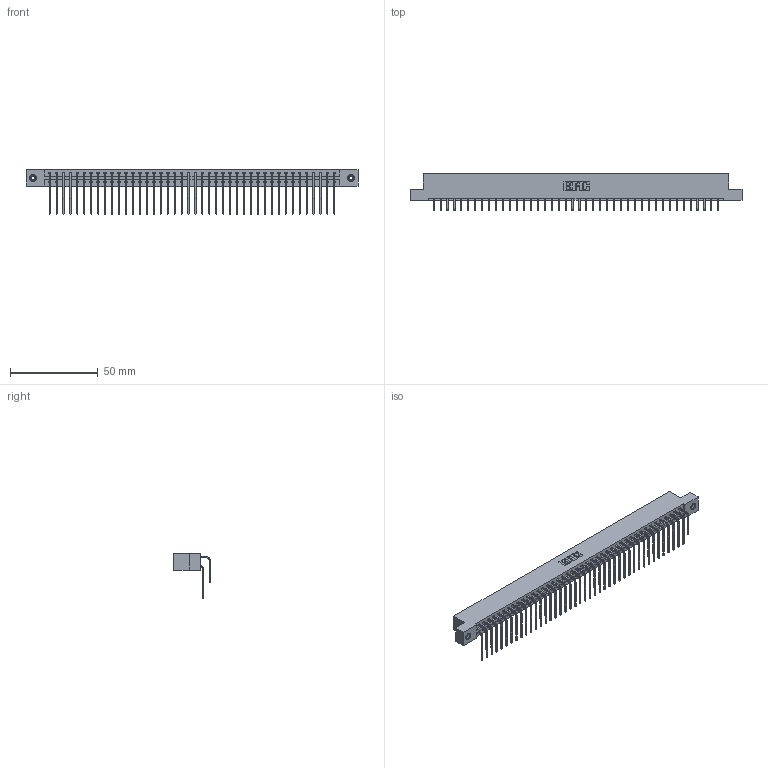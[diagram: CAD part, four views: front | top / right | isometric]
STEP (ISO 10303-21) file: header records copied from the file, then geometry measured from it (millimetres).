
FILE_DESCRIPTION (( 'STEP AP203' ), '1' );
FILE_NAME ('337-084-559-208.STEP', '2019-10-10T14:27:55', ( '' ), ( '' ), 'SwSTEP 2.0', 'SolidWorks 2016', '' );
FILE_SCHEMA (( 'CONFIG_CONTROL_DESIGN' ));
Length unit declared in the file: inch
Products named in the file (5): 345-292-001_559 Tail - 2; 345-250-001_345-250-003-102; 337-084-559-208; 345-292-001_558 559 Tail - 1; 337 Part_Flush Mounting Lugs - 0.156 Dia-TI
Assembly tree (87 placements, depth 2):
  337-084-559-208
    337 Part_Flush Mounting Lugs - 0.156 Dia-TI
    345-292-001_558 559 Tail - 1  x42
    345-292-001_559 Tail - 2  x42
    345-250-001_345-250-003-102  x2
Bounding box: 189.43 x 20.9 x 25.53 mm (x, y, z)
Volume: 20442 mm3; surface area: 25566.8 mm2
Topology: 87 solids, 87 shells, 4878 faces, 14475 edges, 9530 vertices
Faces by surface type: plane 3462, cylinder 1400, cone 12, torus 4
Entity records: 35534 total; most frequent: CARTESIAN_POINT 6012, ORIENTED_EDGE 5890, DIRECTION 5127, EDGE_CURVE 2945, LINE 2757, VECTOR 2757, VERTEX_POINT 1956, AXIS2_PLACEMENT_3D 1185
